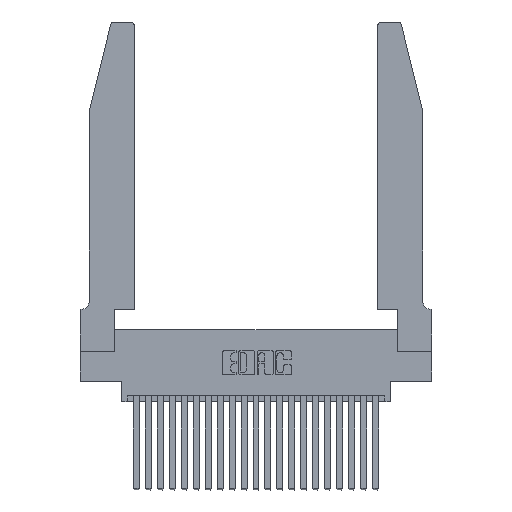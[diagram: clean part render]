
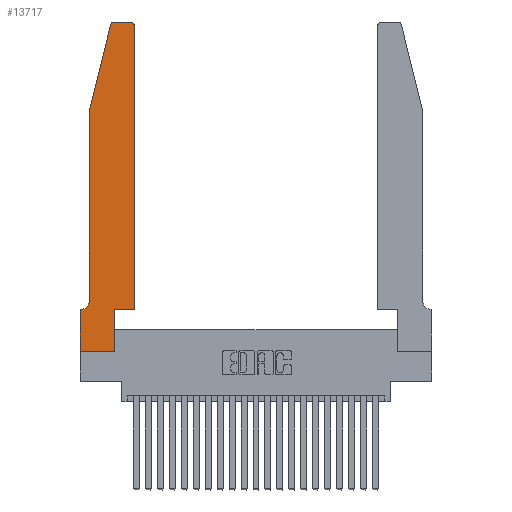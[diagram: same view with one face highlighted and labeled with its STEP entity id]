
A CAD part, top view. The second image highlights one B-rep face of the part: STEP entity #13717.
In plain terms, the highlighted planar face has unit normal (0, 0, 1).
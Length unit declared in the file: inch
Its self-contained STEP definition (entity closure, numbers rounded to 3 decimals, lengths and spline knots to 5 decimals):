
#105 = CIRCLE ( 'NONE', #4258, 0.03 ) ;
#511 = ORIENTED_EDGE ( 'NONE', *, *, #6249, .T. ) ;
#824 = DIRECTION ( 'NONE',  ( -1., 0., 0. ) ) ;
#950 = DIRECTION ( 'NONE',  ( 0., 1., 0. ) ) ;
#955 = CARTESIAN_POINT ( 'NONE',  ( 0.284, 2.75, 0.37 ) ) ;
#1017 = CARTESIAN_POINT ( 'NONE',  ( 0.2865, 0., 0.37 ) ) ;
#1283 = DIRECTION ( 'NONE',  ( -1., 0., 0. ) ) ;
#1315 = CARTESIAN_POINT ( 'NONE',  ( 0.4205, 2.72, 0.37 ) ) ;
#1456 = CARTESIAN_POINT ( 'NONE',  ( 0.0755, 2., 0.37 ) ) ;
#1580 = CARTESIAN_POINT ( 'NONE',  ( 0., 0., 0.37 ) ) ;
#1710 = VERTEX_POINT ( 'NONE', #8902 ) ;
#1915 = DIRECTION ( 'NONE',  ( -1., 0., 0. ) ) ;
#1944 = VERTEX_POINT ( 'NONE', #23780 ) ;
#2218 = ORIENTED_EDGE ( 'NONE', *, *, #3371, .T. ) ;
#2252 = VECTOR ( 'NONE', #950, 39.37008 ) ;
#2709 = EDGE_CURVE ( 'NONE', #21024, #7476, #23585, .T. ) ;
#2786 = DIRECTION ( 'NONE',  ( 0., 0., 1. ) ) ;
#3187 = ORIENTED_EDGE ( 'NONE', *, *, #19110, .T. ) ;
#3194 = DIRECTION ( 'NONE',  ( 1., 0., 0. ) ) ;
#3205 = CARTESIAN_POINT ( 'NONE',  ( 0., 0., 0.37 ) ) ;
#3232 = EDGE_CURVE ( 'NONE', #1944, #21024, #18163, .T. ) ;
#3267 = DIRECTION ( 'NONE',  ( 1., 0., 0. ) ) ;
#3321 = CARTESIAN_POINT ( 'NONE',  ( 0., 0., 0.37 ) ) ;
#3371 = EDGE_CURVE ( 'NONE', #3990, #10125, #11051, .T. ) ;
#3990 = VERTEX_POINT ( 'NONE', #12923 ) ;
#4037 = VECTOR ( 'NONE', #17999, 39.37008 ) ;
#4258 = AXIS2_PLACEMENT_3D ( 'NONE', #13997, #2786, #15796 ) ;
#5064 = CARTESIAN_POINT ( 'NONE',  ( 0.0755, 0.35, 0.37 ) ) ;
#5119 = ORIENTED_EDGE ( 'NONE', *, *, #16011, .T. ) ;
#5142 = CIRCLE ( 'NONE', #9036, 0.03 ) ;
#5699 = CARTESIAN_POINT ( 'NONE',  ( 0.0055, 0.35, 0.37 ) ) ;
#6185 = CARTESIAN_POINT ( 'NONE',  ( 0.4505, 0.35, 0.37 ) ) ;
#6249 = EDGE_CURVE ( 'NONE', #21284, #16181, #7462, .T. ) ;
#6893 = VECTOR ( 'NONE', #21565, 39.37008 ) ;
#6964 = CARTESIAN_POINT ( 'NONE',  ( 0.0755, 2., 0.37 ) ) ;
#7340 = LINE ( 'NONE', #14106, #2252 ) ;
#7369 = VECTOR ( 'NONE', #3194, 39.37008 ) ;
#7462 = LINE ( 'NONE', #6964, #6893 ) ;
#7464 = CARTESIAN_POINT ( 'NONE',  ( 0.0755, 2., 0.37 ) ) ;
#7473 = ORIENTED_EDGE ( 'NONE', *, *, #8194, .T. ) ;
#7476 = VERTEX_POINT ( 'NONE', #1017 ) ;
#8013 = ORIENTED_EDGE ( 'NONE', *, *, #2709, .T. ) ;
#8106 = ORIENTED_EDGE ( 'NONE', *, *, #9705, .T. ) ;
#8194 = EDGE_CURVE ( 'NONE', #13331, #22092, #11748, .T. ) ;
#8445 = VERTEX_POINT ( 'NONE', #5699 ) ;
#8902 = CARTESIAN_POINT ( 'NONE',  ( 0.0755, 0.42, 0.37 ) ) ;
#9016 = VECTOR ( 'NONE', #16525, 39.37008 ) ;
#9036 = AXIS2_PLACEMENT_3D ( 'NONE', #1315, #14435, #3267 ) ;
#9683 = PLANE ( 'NONE',  #18261 ) ;
#9705 = EDGE_CURVE ( 'NONE', #15087, #3990, #5142, .T. ) ;
#10125 = VERTEX_POINT ( 'NONE', #955 ) ;
#10251 = FACE_OUTER_BOUND ( 'NONE', #18187, .T. ) ;
#10369 = DIRECTION ( 'NONE',  ( 0., 1., 0. ) ) ;
#10970 = DIRECTION ( 'NONE',  ( 0., -1., 0. ) ) ;
#11051 = LINE ( 'NONE', #14988, #20689 ) ;
#11181 = CIRCLE ( 'NONE', #14454, 0.07 ) ;
#11542 = DIRECTION ( 'NONE',  ( 1., 0., 0. ) ) ;
#11748 = LINE ( 'NONE', #17994, #7369 ) ;
#12029 = EDGE_CURVE ( 'NONE', #1710, #8445, #11181, .T. ) ;
#12130 = ORIENTED_EDGE ( 'NONE', *, *, #12029, .T. ) ;
#12186 = DIRECTION ( 'NONE',  ( 0., 0., -1. ) ) ;
#12832 = ORIENTED_EDGE ( 'NONE', *, *, #13384, .T. ) ;
#12923 = CARTESIAN_POINT ( 'NONE',  ( 0.4205, 2.75, 0.37 ) ) ;
#13256 = CARTESIAN_POINT ( 'NONE',  ( 0.25487, 2.72718, 0.37 ) ) ;
#13331 = VERTEX_POINT ( 'NONE', #15699 ) ;
#13384 = EDGE_CURVE ( 'NONE', #7476, #13331, #7340, .T. ) ;
#13532 = EDGE_CURVE ( 'NONE', #16181, #1710, #19072, .T. ) ;
#13717 = ADVANCED_FACE ( 'NONE', ( #10251 ), #9683, .T. ) ;
#13989 = LINE ( 'NONE', #21240, #23613 ) ;
#13997 = CARTESIAN_POINT ( 'NONE',  ( 0.284, 2.72, 0.37 ) ) ;
#14106 = CARTESIAN_POINT ( 'NONE',  ( 0.2865, 0.35, 0.37 ) ) ;
#14435 = DIRECTION ( 'NONE',  ( 0., 0., 1. ) ) ;
#14454 = AXIS2_PLACEMENT_3D ( 'NONE', #23029, #12186, #824 ) ;
#14988 = CARTESIAN_POINT ( 'NONE',  ( 0.2605, 2.75, 0.37 ) ) ;
#14998 = CARTESIAN_POINT ( 'NONE',  ( 0.4505, 2.72, 0.37 ) ) ;
#15087 = VERTEX_POINT ( 'NONE', #14998 ) ;
#15699 = CARTESIAN_POINT ( 'NONE',  ( 0.2865, 0.35, 0.37 ) ) ;
#15796 = DIRECTION ( 'NONE',  ( 1., 0., 0. ) ) ;
#16011 = EDGE_CURVE ( 'NONE', #8445, #1944, #24031, .T. ) ;
#16181 = VERTEX_POINT ( 'NONE', #7464 ) ;
#16525 = DIRECTION ( 'NONE',  ( 0., -1., 0. ) ) ;
#17936 = VECTOR ( 'NONE', #10970, 39.37008 ) ;
#17994 = CARTESIAN_POINT ( 'NONE',  ( 0.4505, 0.35, 0.37 ) ) ;
#17999 = DIRECTION ( 'NONE',  ( 1., 0., 0. ) ) ;
#18163 = LINE ( 'NONE', #1580, #9016 ) ;
#18187 = EDGE_LOOP ( 'NONE', ( #2218, #3187, #511, #18735, #12130, #5119, #18522, #8013, #12832, #7473, #19804, #8106 ) ) ;
#18261 = AXIS2_PLACEMENT_3D ( 'NONE', #18667, #22392, #11542 ) ;
#18522 = ORIENTED_EDGE ( 'NONE', *, *, #3232, .T. ) ;
#18667 = CARTESIAN_POINT ( 'NONE',  ( 0., 0.35, 0.37 ) ) ;
#18735 = ORIENTED_EDGE ( 'NONE', *, *, #13532, .T. ) ;
#19072 = LINE ( 'NONE', #1456, #17936 ) ;
#19110 = EDGE_CURVE ( 'NONE', #10125, #21284, #105, .T. ) ;
#19125 = EDGE_CURVE ( 'NONE', #22092, #15087, #13989, .T. ) ;
#19212 = VECTOR ( 'NONE', #1283, 39.37008 ) ;
#19804 = ORIENTED_EDGE ( 'NONE', *, *, #19125, .T. ) ;
#20689 = VECTOR ( 'NONE', #1915, 39.37008 ) ;
#21024 = VERTEX_POINT ( 'NONE', #3205 ) ;
#21240 = CARTESIAN_POINT ( 'NONE',  ( 0.4505, 0.35, 0.37 ) ) ;
#21284 = VERTEX_POINT ( 'NONE', #13256 ) ;
#21565 = DIRECTION ( 'NONE',  ( -0.239, -0.971, 0. ) ) ;
#22092 = VERTEX_POINT ( 'NONE', #6185 ) ;
#22392 = DIRECTION ( 'NONE',  ( 0., 0., 1. ) ) ;
#23029 = CARTESIAN_POINT ( 'NONE',  ( 0.0055, 0.42, 0.37 ) ) ;
#23585 = LINE ( 'NONE', #3321, #4037 ) ;
#23613 = VECTOR ( 'NONE', #10369, 39.37008 ) ;
#23780 = CARTESIAN_POINT ( 'NONE',  ( 0., 0.35, 0.37 ) ) ;
#24031 = LINE ( 'NONE', #5064, #19212 ) ;
